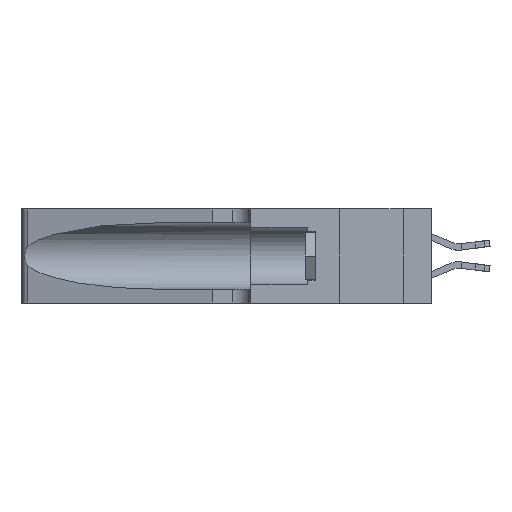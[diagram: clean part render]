
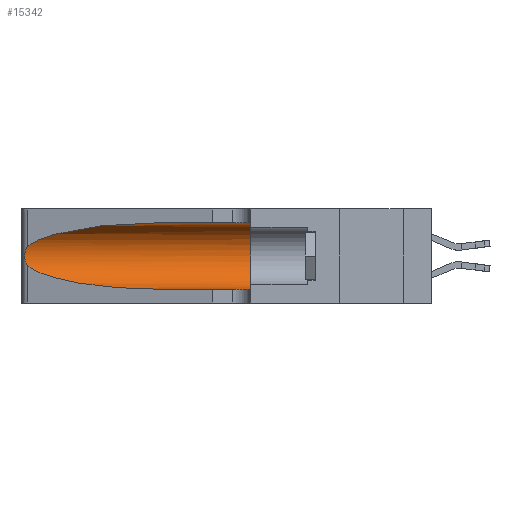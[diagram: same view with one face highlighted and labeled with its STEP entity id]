
A CAD part, left-side view. The second image highlights one B-rep face of the part: STEP entity #15342.
In plain terms, the highlighted cylindrical face has radius 3.308 mm (diameter 6.617 mm), a partial arc.
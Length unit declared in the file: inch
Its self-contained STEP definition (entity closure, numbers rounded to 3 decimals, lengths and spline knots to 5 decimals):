
#1194 = EDGE_CURVE ( 'NONE', #7706, #17028, #10243, .T. ) ;
#1847 = CARTESIAN_POINT ( 'NONE',  ( 0.1305, 1.61858, 0.31525 ) ) ;
#2070 = LINE ( 'NONE', #1847, #14574 ) ;
#2297 = CARTESIAN_POINT ( 'NONE',  ( 0.1305, 0.72297, 0.05475 ) ) ;
#2751 = ORIENTED_EDGE ( 'NONE', *, *, #14600, .T. ) ;
#3729 = VERTEX_POINT ( 'NONE', #27267 ) ;
#3738 = ORIENTED_EDGE ( 'NONE', *, *, #7952, .F. ) ;
#4446 = CARTESIAN_POINT ( 'NONE',  ( 0.25555, 1.22994, 0.2215 ) ) ;
#4649 = CARTESIAN_POINT ( 'NONE',  ( 0.26075, 1.23896, 0.178 ) ) ;
#4875 = CARTESIAN_POINT ( 'NONE',  ( 0.2373, 1.15595, 0.28018 ) ) ;
#5435 = AXIS2_PLACEMENT_3D ( 'NONE', #21305, #21057, #23624 ) ;
#5763 = CARTESIAN_POINT ( 'NONE',  ( 0.1305, 1.61858, 0.05475 ) ) ;
#5766 = EDGE_CURVE ( 'NONE', #31603, #3729, #14715, .T. ) ;
#5771 = CARTESIAN_POINT ( 'NONE',  ( 0.1305, 0.72297, 0.05475 ) ) ;
#6306 = DIRECTION ( 'NONE',  ( 0., 0., 1. ) ) ;
#7258 = CARTESIAN_POINT ( 'NONE',  ( 0.26017, 1.23833, 0.17102 ) ) ;
#7363 = CARTESIAN_POINT ( 'NONE',  ( 0.26075, 1.23896, 0.19203 ) ) ;
#7706 = VERTEX_POINT ( 'NONE', #8479 ) ;
#7902 = VERTEX_POINT ( 'NONE', #13397 ) ;
#7952 = EDGE_CURVE ( 'NONE', #7902, #14950, #2070, .T. ) ;
#8479 = CARTESIAN_POINT ( 'NONE',  ( 0.25487, 1.22718, 0.22369 ) ) ;
#9627 = CARTESIAN_POINT ( 'NONE',  ( 0.18966, 0.96281, 0.05475 ) ) ;
#10243 = B_SPLINE_CURVE_WITH_KNOTS ( 'NONE', 3,
 ( #17077, #4446, #19376, #19598, #32157, #22221, #7363, #4649, #7258, #14780, #17182, #14467, #24743, #26968 ),
 .UNSPECIFIED., .F., .F.,
 ( 4, 2, 2, 2, 2, 2, 4 ),
 ( 0., 0.00027, 0.00053, 0.00107, 0.0016, 0.00187, 0.00214 ),
 .UNSPECIFIED. ) ;
#12585 = ORIENTED_EDGE ( 'NONE', *, *, #22843, .F. ) ;
#13397 = CARTESIAN_POINT ( 'NONE',  ( 0.1305, 0.72297, 0.31525 ) ) ;
#13755 = DIRECTION ( 'NONE',  ( 0., -1., 0. ) ) ;
#13900 = CARTESIAN_POINT ( 'NONE',  ( 0.1305, 0.35, 0.31525 ) ) ;
#14145 = CIRCLE ( 'NONE', #20634, 0.13025 ) ;
#14417 = DIRECTION ( 'NONE',  ( 0., -1., 0. ) ) ;
#14467 = CARTESIAN_POINT ( 'NONE',  ( 0.25639, 1.23186, 0.15144 ) ) ;
#14574 = VECTOR ( 'NONE', #14417, 39.37008 ) ;
#14600 = EDGE_CURVE ( 'NONE', #17028, #31603, #26743, .T. ) ;
#14698 = CARTESIAN_POINT ( 'NONE',  ( 0.1305, 0.72297, 0.31525 ) ) ;
#14715 = LINE ( 'NONE', #5763, #28824 ) ;
#14780 = CARTESIAN_POINT ( 'NONE',  ( 0.25856, 1.23593, 0.16098 ) ) ;
#14950 = VERTEX_POINT ( 'NONE', #13900 ) ;
#15342 = ADVANCED_FACE ( 'NONE', ( #21774 ), #29251, .F. ) ;
#17028 = VERTEX_POINT ( 'NONE', #19798 ) ;
#17077 = CARTESIAN_POINT ( 'NONE',  ( 0.25487, 1.22718, 0.22369 ) ) ;
#17182 = CARTESIAN_POINT ( 'NONE',  ( 0.25789, 1.23486, 0.15765 ) ) ;
#19315 = EDGE_CURVE ( 'NONE', #7902, #7706, #22833, .T. ) ;
#19376 = CARTESIAN_POINT ( 'NONE',  ( 0.25639, 1.23184, 0.21858 ) ) ;
#19598 = CARTESIAN_POINT ( 'NONE',  ( 0.25787, 1.23484, 0.2124 ) ) ;
#19798 = CARTESIAN_POINT ( 'NONE',  ( 0.25487, 1.22718, 0.14631 ) ) ;
#19831 = CARTESIAN_POINT ( 'NONE',  ( 0.25487, 1.22718, 0.22369 ) ) ;
#20634 = AXIS2_PLACEMENT_3D ( 'NONE', #26438, #31227, #6306 ) ;
#21057 = DIRECTION ( 'NONE',  ( 0., -1., 0. ) ) ;
#21190 = CARTESIAN_POINT ( 'NONE',  ( 0.2373, 1.15595, 0.08982 ) ) ;
#21305 = CARTESIAN_POINT ( 'NONE',  ( 0.1305, 1.61858, 0.185 ) ) ;
#21774 = FACE_OUTER_BOUND ( 'NONE', #27600, .T. ) ;
#22144 = CARTESIAN_POINT ( 'NONE',  ( 0.18966, 0.96281, 0.31525 ) ) ;
#22221 = CARTESIAN_POINT ( 'NONE',  ( 0.26018, 1.23835, 0.19895 ) ) ;
#22833 =( BOUNDED_CURVE ( )  B_SPLINE_CURVE ( 3, ( #14698, #22144, #4875, #19831 ),
 .UNSPECIFIED., .F., .T. ) 
 B_SPLINE_CURVE_WITH_KNOTS ( ( 4, 4 ),
 ( 1.5708, 2.84003 ),
 .UNSPECIFIED. ) 
 CURVE ( )  GEOMETRIC_REPRESENTATION_ITEM ( )  RATIONAL_B_SPLINE_CURVE ( ( 1., 0.87, 0.87, 1. ) ) 
 REPRESENTATION_ITEM ( '' )  );
#22843 = EDGE_CURVE ( 'NONE', #14950, #3729, #14145, .T. ) ;
#23624 = DIRECTION ( 'NONE',  ( 0., 0., -1. ) ) ;
#24743 = CARTESIAN_POINT ( 'NONE',  ( 0.25555, 1.22993, 0.14849 ) ) ;
#26438 = CARTESIAN_POINT ( 'NONE',  ( 0.1305, 0.35, 0.185 ) ) ;
#26743 =( BOUNDED_CURVE ( )  B_SPLINE_CURVE ( 3, ( #29226, #21190, #9627, #2297 ),
 .UNSPECIFIED., .F., .T. ) 
 B_SPLINE_CURVE_WITH_KNOTS ( ( 4, 4 ),
 ( 3.44316, 4.71239 ),
 .UNSPECIFIED. ) 
 CURVE ( )  GEOMETRIC_REPRESENTATION_ITEM ( )  RATIONAL_B_SPLINE_CURVE ( ( 1., 0.87, 0.87, 1. ) ) 
 REPRESENTATION_ITEM ( '' )  );
#26968 = CARTESIAN_POINT ( 'NONE',  ( 0.25487, 1.22718, 0.14631 ) ) ;
#27267 = CARTESIAN_POINT ( 'NONE',  ( 0.1305, 0.35, 0.05475 ) ) ;
#27600 = EDGE_LOOP ( 'NONE', ( #29795, #32195, #2751, #31902, #12585, #3738 ) ) ;
#28824 = VECTOR ( 'NONE', #13755, 39.37008 ) ;
#29226 = CARTESIAN_POINT ( 'NONE',  ( 0.25487, 1.22718, 0.14631 ) ) ;
#29251 = CYLINDRICAL_SURFACE ( 'NONE', #5435, 0.13025 ) ;
#29795 = ORIENTED_EDGE ( 'NONE', *, *, #19315, .T. ) ;
#31227 = DIRECTION ( 'NONE',  ( 0., 1., 0. ) ) ;
#31603 = VERTEX_POINT ( 'NONE', #5771 ) ;
#31902 = ORIENTED_EDGE ( 'NONE', *, *, #5766, .T. ) ;
#32157 = CARTESIAN_POINT ( 'NONE',  ( 0.25854, 1.2359, 0.20912 ) ) ;
#32195 = ORIENTED_EDGE ( 'NONE', *, *, #1194, .T. ) ;
